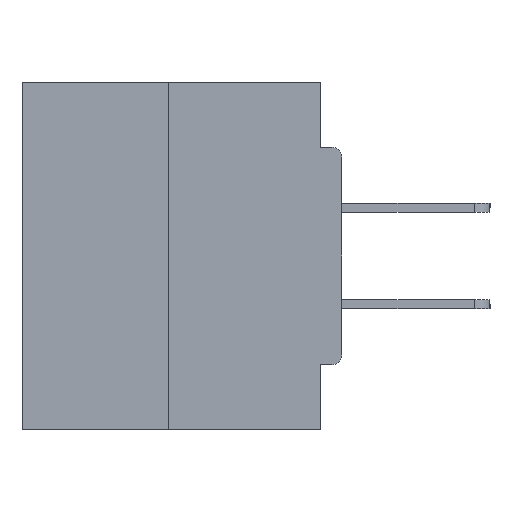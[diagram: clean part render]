
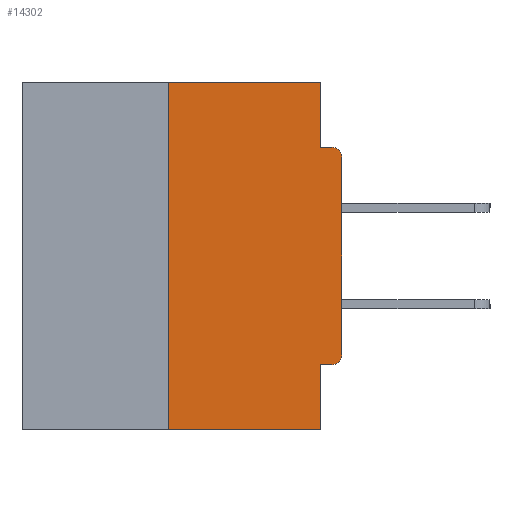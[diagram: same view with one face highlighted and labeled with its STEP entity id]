
A CAD part, left-side view. The second image highlights one B-rep face of the part: STEP entity #14302.
In plain terms, the highlighted planar face has unit normal (-1, 0, 0).
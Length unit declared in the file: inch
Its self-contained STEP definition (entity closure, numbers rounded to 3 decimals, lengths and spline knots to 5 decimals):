
#615 = ORIENTED_EDGE ( 'NONE', *, *, #35923, .T. ) ;
#641 = PLANE ( 'NONE',  #27690 ) ;
#898 = CARTESIAN_POINT ( 'NONE',  ( 0., 0.25, 0. ) ) ;
#973 = CARTESIAN_POINT ( 'NONE',  ( 0., 0.031, 0. ) ) ;
#1171 = DIRECTION ( 'NONE',  ( 0., 0., -1. ) ) ;
#2404 = DIRECTION ( 'NONE',  ( -1., 0., 0. ) ) ;
#2443 = CARTESIAN_POINT ( 'NONE',  ( 0., 0.015, -0.0935 ) ) ;
#2682 = EDGE_CURVE ( 'NONE', #36122, #12623, #32153, .T. ) ;
#2705 = LINE ( 'NONE', #35429, #5834 ) ;
#2751 = VERTEX_POINT ( 'NONE', #13237 ) ;
#2911 = DIRECTION ( 'NONE',  ( 0., 0., -1. ) ) ;
#3450 = ORIENTED_EDGE ( 'NONE', *, *, #10273, .F. ) ;
#3500 = EDGE_CURVE ( 'NONE', #33849, #12623, #4977, .T. ) ;
#3787 = EDGE_CURVE ( 'NONE', #26754, #2751, #9236, .T. ) ;
#4184 = ORIENTED_EDGE ( 'NONE', *, *, #3787, .T. ) ;
#4486 = VERTEX_POINT ( 'NONE', #15365 ) ;
#4927 = EDGE_LOOP ( 'NONE', ( #3450, #10807, #28088, #26378, #26375, #4184, #615, #31714, #22636, #21545 ) ) ;
#4938 = VECTOR ( 'NONE', #8483, 39.37008 ) ;
#4977 = LINE ( 'NONE', #34778, #8523 ) ;
#5826 = VERTEX_POINT ( 'NONE', #13408 ) ;
#5834 = VECTOR ( 'NONE', #23883, 39.37008 ) ;
#6461 = LINE ( 'NONE', #28169, #17837 ) ;
#6849 = EDGE_CURVE ( 'NONE', #4486, #36144, #23488, .T. ) ;
#6933 = DIRECTION ( 'NONE',  ( 0., -1., 0. ) ) ;
#7592 = DIRECTION ( 'NONE',  ( 0., 0., -1. ) ) ;
#8483 = DIRECTION ( 'NONE',  ( 0., 0., 1. ) ) ;
#8523 = VECTOR ( 'NONE', #6933, 39.37008 ) ;
#9236 = CIRCLE ( 'NONE', #24639, 0.015 ) ;
#10119 = VERTEX_POINT ( 'NONE', #973 ) ;
#10273 = EDGE_CURVE ( 'NONE', #25985, #10119, #2705, .T. ) ;
#10807 = ORIENTED_EDGE ( 'NONE', *, *, #15782, .F. ) ;
#12623 = VERTEX_POINT ( 'NONE', #2443 ) ;
#13237 = CARTESIAN_POINT ( 'NONE',  ( 0., 0., -0.3915 ) ) ;
#13358 = CARTESIAN_POINT ( 'NONE',  ( 0., 0.015, -0.1085 ) ) ;
#13408 = CARTESIAN_POINT ( 'NONE',  ( 0., 0.25, -0.5 ) ) ;
#13590 = DIRECTION ( 'NONE',  ( 0., 0., -1. ) ) ;
#14045 = VECTOR ( 'NONE', #27702, 39.37008 ) ;
#14302 = ADVANCED_FACE ( 'NONE', ( #15403 ), #641, .F. ) ;
#14546 = EDGE_CURVE ( 'NONE', #10119, #33849, #22768, .T. ) ;
#14756 = CARTESIAN_POINT ( 'NONE',  ( 0., 0.25, 0. ) ) ;
#15365 = CARTESIAN_POINT ( 'NONE',  ( 0., 0.031, -0.4065 ) ) ;
#15403 = FACE_OUTER_BOUND ( 'NONE', #4927, .T. ) ;
#15668 = CARTESIAN_POINT ( 'NONE',  ( 0., 0.031, -0.5 ) ) ;
#15782 = EDGE_CURVE ( 'NONE', #5826, #25985, #29673, .T. ) ;
#15832 = VECTOR ( 'NONE', #13590, 39.37008 ) ;
#17396 = DIRECTION ( 'NONE',  ( 0., -1., 0. ) ) ;
#17837 = VECTOR ( 'NONE', #17396, 39.37008 ) ;
#17958 = DIRECTION ( 'NONE',  ( -1., 0., 0. ) ) ;
#18497 = EDGE_CURVE ( 'NONE', #5826, #36144, #6461, .T. ) ;
#18596 = CARTESIAN_POINT ( 'NONE',  ( 0., 0., -0.1085 ) ) ;
#19470 = DIRECTION ( 'NONE',  ( 0., 1., 0. ) ) ;
#20248 = DIRECTION ( 'NONE',  ( 1., 0., 0. ) ) ;
#20981 = CARTESIAN_POINT ( 'NONE',  ( 0., 0.015, -0.3915 ) ) ;
#21545 = ORIENTED_EDGE ( 'NONE', *, *, #14546, .F. ) ;
#21791 = VECTOR ( 'NONE', #19470, 39.37008 ) ;
#22111 = CARTESIAN_POINT ( 'NONE',  ( 0., 0., -0.4065 ) ) ;
#22636 = ORIENTED_EDGE ( 'NONE', *, *, #3500, .F. ) ;
#22768 = LINE ( 'NONE', #24622, #15832 ) ;
#22775 = EDGE_CURVE ( 'NONE', #26754, #4486, #26185, .T. ) ;
#23488 = LINE ( 'NONE', #31218, #29993 ) ;
#23883 = DIRECTION ( 'NONE',  ( 0., -1., 0. ) ) ;
#24622 = CARTESIAN_POINT ( 'NONE',  ( 0., 0.031, 0. ) ) ;
#24639 = AXIS2_PLACEMENT_3D ( 'NONE', #20981, #17958, #1171 ) ;
#24855 = AXIS2_PLACEMENT_3D ( 'NONE', #13358, #2404, #7592 ) ;
#25403 = CARTESIAN_POINT ( 'NONE',  ( 0., 0., 0. ) ) ;
#25985 = VERTEX_POINT ( 'NONE', #898 ) ;
#26185 = LINE ( 'NONE', #22111, #21791 ) ;
#26375 = ORIENTED_EDGE ( 'NONE', *, *, #22775, .F. ) ;
#26378 = ORIENTED_EDGE ( 'NONE', *, *, #6849, .F. ) ;
#26754 = VERTEX_POINT ( 'NONE', #34985 ) ;
#27690 = AXIS2_PLACEMENT_3D ( 'NONE', #28860, #20248, #28603 ) ;
#27702 = DIRECTION ( 'NONE',  ( 0., 0., 1. ) ) ;
#28088 = ORIENTED_EDGE ( 'NONE', *, *, #18497, .T. ) ;
#28169 = CARTESIAN_POINT ( 'NONE',  ( 0., 0.46, -0.5 ) ) ;
#28603 = DIRECTION ( 'NONE',  ( 0., 0., -1. ) ) ;
#28860 = CARTESIAN_POINT ( 'NONE',  ( 0., 0.46, 0. ) ) ;
#29673 = LINE ( 'NONE', #14756, #14045 ) ;
#29993 = VECTOR ( 'NONE', #2911, 39.37008 ) ;
#30694 = LINE ( 'NONE', #25403, #4938 ) ;
#31218 = CARTESIAN_POINT ( 'NONE',  ( 0., 0.031, -0.5 ) ) ;
#31714 = ORIENTED_EDGE ( 'NONE', *, *, #2682, .T. ) ;
#32153 = CIRCLE ( 'NONE', #24855, 0.015 ) ;
#33068 = CARTESIAN_POINT ( 'NONE',  ( 0., 0.031, -0.0935 ) ) ;
#33849 = VERTEX_POINT ( 'NONE', #33068 ) ;
#34778 = CARTESIAN_POINT ( 'NONE',  ( 0., 0., -0.0935 ) ) ;
#34985 = CARTESIAN_POINT ( 'NONE',  ( 0., 0.015, -0.4065 ) ) ;
#35429 = CARTESIAN_POINT ( 'NONE',  ( 0., 0.46, 0. ) ) ;
#35923 = EDGE_CURVE ( 'NONE', #2751, #36122, #30694, .T. ) ;
#36122 = VERTEX_POINT ( 'NONE', #18596 ) ;
#36144 = VERTEX_POINT ( 'NONE', #15668 ) ;
